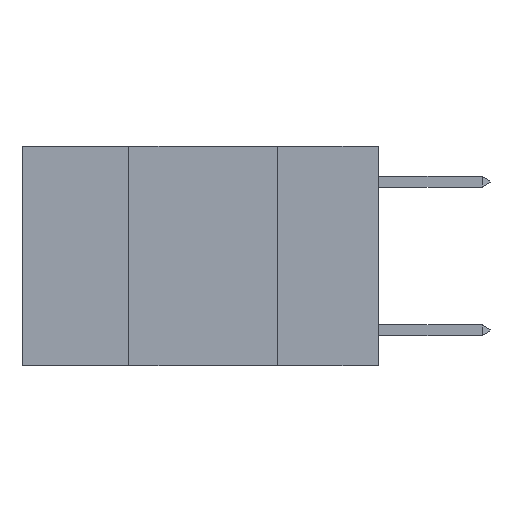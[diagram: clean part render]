
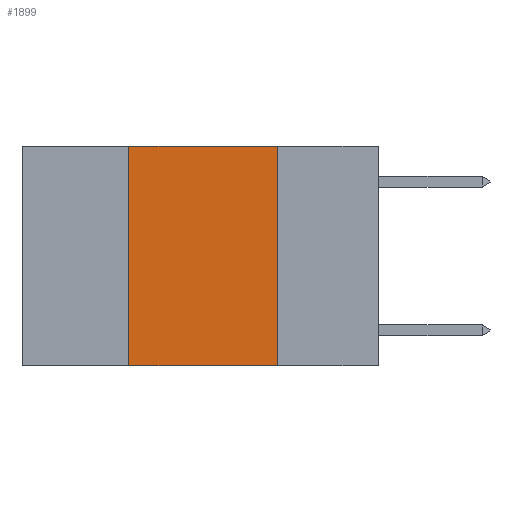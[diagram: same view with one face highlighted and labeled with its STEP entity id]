
A CAD part, left-side view. The second image highlights one B-rep face of the part: STEP entity #1899.
In plain terms, the highlighted planar face has unit normal (-1, 0, 0).
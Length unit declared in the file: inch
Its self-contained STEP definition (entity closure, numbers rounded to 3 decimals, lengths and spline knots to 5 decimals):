
#288 = VERTEX_POINT ( 'NONE', #1743 ) ;
#568 = AXIS2_PLACEMENT_3D ( 'NONE', #2479, #11208, #14557 ) ;
#634 = VERTEX_POINT ( 'NONE', #21862 ) ;
#951 = VECTOR ( 'NONE', #17130, 39.37008 ) ;
#1743 = CARTESIAN_POINT ( 'NONE',  ( 0., 0.42, 0. ) ) ;
#1899 = ADVANCED_FACE ( 'NONE', ( #21148 ), #7498, .F. ) ;
#2049 = VECTOR ( 'NONE', #2859, 39.37008 ) ;
#2060 = LINE ( 'NONE', #3524, #4958 ) ;
#2479 = CARTESIAN_POINT ( 'NONE',  ( 0., 0.6, 0. ) ) ;
#2627 = ORIENTED_EDGE ( 'NONE', *, *, #2665, .T. ) ;
#2665 = EDGE_CURVE ( 'NONE', #634, #21869, #2060, .T. ) ;
#2859 = DIRECTION ( 'NONE',  ( 0., 0., -1. ) ) ;
#3188 = LINE ( 'NONE', #8328, #17590 ) ;
#3524 = CARTESIAN_POINT ( 'NONE',  ( 0., 0.6, -0.37 ) ) ;
#4555 = EDGE_CURVE ( 'NONE', #288, #10822, #15561, .T. ) ;
#4958 = VECTOR ( 'NONE', #13932, 39.37008 ) ;
#5172 = CARTESIAN_POINT ( 'NONE',  ( 0., 0.6, 0. ) ) ;
#6863 = ORIENTED_EDGE ( 'NONE', *, *, #7464, .F. ) ;
#7148 = CARTESIAN_POINT ( 'NONE',  ( 0., 0.17, 0. ) ) ;
#7464 = EDGE_CURVE ( 'NONE', #10822, #21869, #14721, .T. ) ;
#7498 = PLANE ( 'NONE',  #568 ) ;
#7986 = DIRECTION ( 'NONE',  ( 0., 0., 1. ) ) ;
#8328 = CARTESIAN_POINT ( 'NONE',  ( 0., 0.42, 0. ) ) ;
#10822 = VERTEX_POINT ( 'NONE', #7148 ) ;
#11208 = DIRECTION ( 'NONE',  ( 1., 0., 0. ) ) ;
#11902 = EDGE_CURVE ( 'NONE', #634, #288, #3188, .T. ) ;
#13047 = CARTESIAN_POINT ( 'NONE',  ( 0., 0.17, 0. ) ) ;
#13816 = CARTESIAN_POINT ( 'NONE',  ( 0., 0.17, -0.37 ) ) ;
#13932 = DIRECTION ( 'NONE',  ( 0., -1., 0. ) ) ;
#14557 = DIRECTION ( 'NONE',  ( 0., 0., -1. ) ) ;
#14721 = LINE ( 'NONE', #13047, #2049 ) ;
#15561 = LINE ( 'NONE', #5172, #951 ) ;
#17130 = DIRECTION ( 'NONE',  ( 0., -1., 0. ) ) ;
#17590 = VECTOR ( 'NONE', #7986, 39.37008 ) ;
#20435 = ORIENTED_EDGE ( 'NONE', *, *, #4555, .F. ) ;
#20749 = ORIENTED_EDGE ( 'NONE', *, *, #11902, .F. ) ;
#21148 = FACE_OUTER_BOUND ( 'NONE', #21201, .T. ) ;
#21201 = EDGE_LOOP ( 'NONE', ( #6863, #20435, #20749, #2627 ) ) ;
#21862 = CARTESIAN_POINT ( 'NONE',  ( 0., 0.42, -0.37 ) ) ;
#21869 = VERTEX_POINT ( 'NONE', #13816 ) ;
